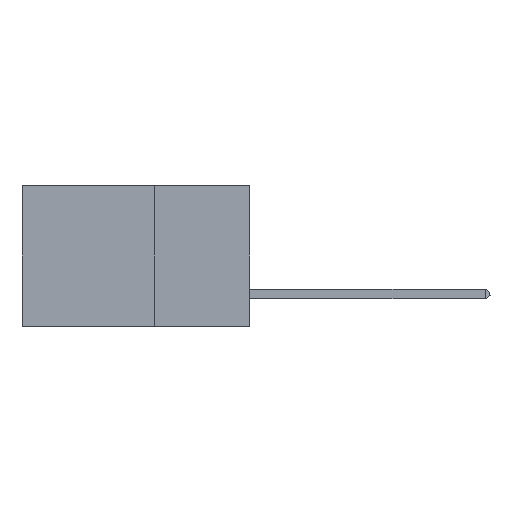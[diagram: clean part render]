
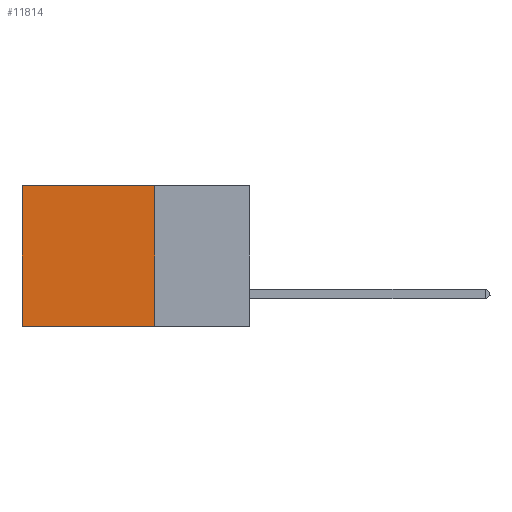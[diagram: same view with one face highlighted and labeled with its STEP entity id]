
A CAD part, left-side view. The second image highlights one B-rep face of the part: STEP entity #11814.
In plain terms, the highlighted planar face has unit normal (-1, 0, 0).
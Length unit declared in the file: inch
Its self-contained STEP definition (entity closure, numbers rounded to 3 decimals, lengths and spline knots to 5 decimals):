
#911 = VECTOR ( 'NONE', #14880, 39.37008 ) ;
#1024 = EDGE_CURVE ( 'NONE', #19863, #22463, #10645, .T. ) ;
#2103 = ORIENTED_EDGE ( 'NONE', *, *, #16418, .T. ) ;
#3090 = CARTESIAN_POINT ( 'NONE',  ( 0.2875, 0.25, 0. ) ) ;
#3778 = ORIENTED_EDGE ( 'NONE', *, *, #10010, .T. ) ;
#4165 = PLANE ( 'NONE',  #4650 ) ;
#4650 = AXIS2_PLACEMENT_3D ( 'NONE', #11289, #13237, #15016 ) ;
#5100 = LINE ( 'NONE', #15585, #21700 ) ;
#5120 = ORIENTED_EDGE ( 'NONE', *, *, #1024, .F. ) ;
#6032 = VERTEX_POINT ( 'NONE', #21163 ) ;
#6173 = FACE_OUTER_BOUND ( 'NONE', #17515, .T. ) ;
#7084 = VECTOR ( 'NONE', #21720, 39.37008 ) ;
#7546 = VECTOR ( 'NONE', #15301, 39.37008 ) ;
#8344 = CARTESIAN_POINT ( 'NONE',  ( 0.2875, 0.25, -0.37 ) ) ;
#9336 = CARTESIAN_POINT ( 'NONE',  ( 0.2875, 0.25, -0.37 ) ) ;
#10010 = EDGE_CURVE ( 'NONE', #19438, #6032, #5100, .T. ) ;
#10645 = LINE ( 'NONE', #9336, #7084 ) ;
#11289 = CARTESIAN_POINT ( 'NONE',  ( 0.2875, 0.25, 0. ) ) ;
#11386 = CARTESIAN_POINT ( 'NONE',  ( 0.2875, 0.6, -0.37 ) ) ;
#11814 = ADVANCED_FACE ( 'NONE', ( #6173 ), #4165, .F. ) ;
#12313 = EDGE_CURVE ( 'NONE', #19438, #19863, #21662, .T. ) ;
#13237 = DIRECTION ( 'NONE',  ( 1., 0., 0. ) ) ;
#13977 = LINE ( 'NONE', #19772, #911 ) ;
#14880 = DIRECTION ( 'NONE',  ( 0., 0., -1. ) ) ;
#15016 = DIRECTION ( 'NONE',  ( 0., 0., -1. ) ) ;
#15301 = DIRECTION ( 'NONE',  ( 0., 0., -1. ) ) ;
#15585 = CARTESIAN_POINT ( 'NONE',  ( 0.2875, 0.25, 0. ) ) ;
#16418 = EDGE_CURVE ( 'NONE', #6032, #22463, #13977, .T. ) ;
#17515 = EDGE_LOOP ( 'NONE', ( #2103, #5120, #22359, #3778 ) ) ;
#18777 = CARTESIAN_POINT ( 'NONE',  ( 0.2875, 0.25, 0. ) ) ;
#19000 = DIRECTION ( 'NONE',  ( 0., 1., 0. ) ) ;
#19438 = VERTEX_POINT ( 'NONE', #3090 ) ;
#19772 = CARTESIAN_POINT ( 'NONE',  ( 0.2875, 0.6, 0. ) ) ;
#19863 = VERTEX_POINT ( 'NONE', #8344 ) ;
#21163 = CARTESIAN_POINT ( 'NONE',  ( 0.2875, 0.6, 0. ) ) ;
#21662 = LINE ( 'NONE', #18777, #7546 ) ;
#21700 = VECTOR ( 'NONE', #19000, 39.37008 ) ;
#21720 = DIRECTION ( 'NONE',  ( 0., 1., 0. ) ) ;
#22359 = ORIENTED_EDGE ( 'NONE', *, *, #12313, .F. ) ;
#22463 = VERTEX_POINT ( 'NONE', #11386 ) ;
